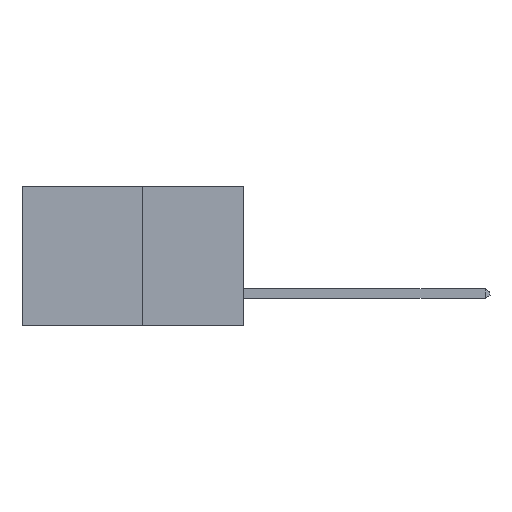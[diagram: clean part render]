
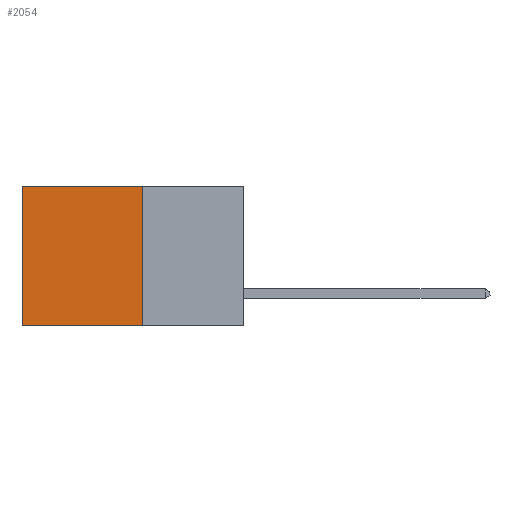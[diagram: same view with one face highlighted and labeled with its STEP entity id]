
A CAD part, left-side view. The second image highlights one B-rep face of the part: STEP entity #2054.
In plain terms, the highlighted planar face has unit normal (-1, 0, 0).
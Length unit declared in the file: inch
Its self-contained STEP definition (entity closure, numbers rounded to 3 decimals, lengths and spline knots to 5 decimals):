
#268 = CARTESIAN_POINT ( 'NONE',  ( 0.277, 0.59, 0. ) ) ;
#414 = EDGE_CURVE ( 'NONE', #2269, #11813, #3332, .T. ) ;
#466 = DIRECTION ( 'NONE',  ( 0., 0., -1. ) ) ;
#1180 = VECTOR ( 'NONE', #466, 39.37008 ) ;
#1765 = ORIENTED_EDGE ( 'NONE', *, *, #11740, .F. ) ;
#2054 = ADVANCED_FACE ( 'NONE', ( #6898 ), #11817, .F. ) ;
#2269 = VERTEX_POINT ( 'NONE', #8996 ) ;
#2298 = DIRECTION ( 'NONE',  ( 0., 0., -1. ) ) ;
#2674 = ORIENTED_EDGE ( 'NONE', *, *, #6995, .T. ) ;
#2815 = LINE ( 'NONE', #4926, #10935 ) ;
#3160 = EDGE_LOOP ( 'NONE', ( #2674, #1765, #12111, #7967 ) ) ;
#3332 = LINE ( 'NONE', #4265, #11753 ) ;
#3892 = DIRECTION ( 'NONE',  ( 0., 1., 0. ) ) ;
#4015 = DIRECTION ( 'NONE',  ( 1., 0., 0. ) ) ;
#4265 = CARTESIAN_POINT ( 'NONE',  ( 0.277, 0.27, -0.37 ) ) ;
#4926 = CARTESIAN_POINT ( 'NONE',  ( 0.277, 0.27, -0.37 ) ) ;
#5611 = CARTESIAN_POINT ( 'NONE',  ( 0.277, 0.27, -0.37 ) ) ;
#6059 = DIRECTION ( 'NONE',  ( 0., 0., -1. ) ) ;
#6538 = DIRECTION ( 'NONE',  ( 0., 1., 0. ) ) ;
#6898 = FACE_OUTER_BOUND ( 'NONE', #3160, .T. ) ;
#6995 = EDGE_CURVE ( 'NONE', #8620, #9443, #9708, .T. ) ;
#7401 = EDGE_CURVE ( 'NONE', #2269, #8620, #13540, .T. ) ;
#7811 = CARTESIAN_POINT ( 'NONE',  ( 0.277, 0.59, -0.37 ) ) ;
#7967 = ORIENTED_EDGE ( 'NONE', *, *, #7401, .T. ) ;
#8053 = VECTOR ( 'NONE', #6538, 39.37008 ) ;
#8620 = VERTEX_POINT ( 'NONE', #268 ) ;
#8996 = CARTESIAN_POINT ( 'NONE',  ( 0.277, 0.27, 0. ) ) ;
#9443 = VERTEX_POINT ( 'NONE', #7811 ) ;
#9708 = LINE ( 'NONE', #12145, #1180 ) ;
#10063 = AXIS2_PLACEMENT_3D ( 'NONE', #5611, #4015, #6059 ) ;
#10935 = VECTOR ( 'NONE', #3892, 39.37008 ) ;
#11339 = CARTESIAN_POINT ( 'NONE',  ( 0.277, 0.27, -0.37 ) ) ;
#11740 = EDGE_CURVE ( 'NONE', #11813, #9443, #2815, .T. ) ;
#11753 = VECTOR ( 'NONE', #2298, 39.37008 ) ;
#11772 = CARTESIAN_POINT ( 'NONE',  ( 0.277, 0.27, 0. ) ) ;
#11813 = VERTEX_POINT ( 'NONE', #11339 ) ;
#11817 = PLANE ( 'NONE',  #10063 ) ;
#12111 = ORIENTED_EDGE ( 'NONE', *, *, #414, .F. ) ;
#12145 = CARTESIAN_POINT ( 'NONE',  ( 0.277, 0.59, -0.37 ) ) ;
#13540 = LINE ( 'NONE', #11772, #8053 ) ;
